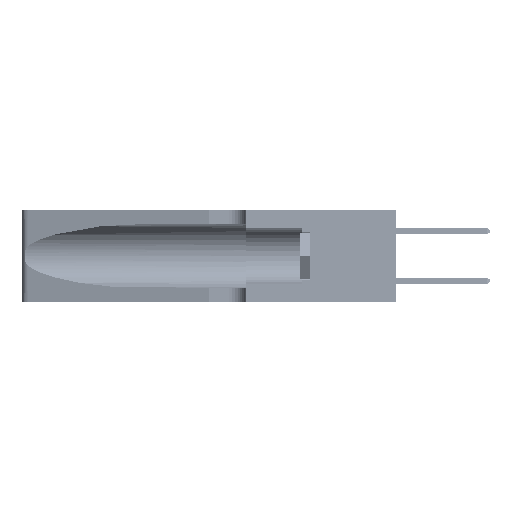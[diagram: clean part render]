
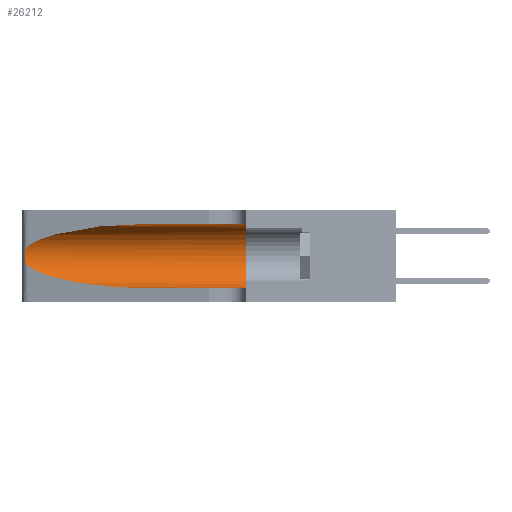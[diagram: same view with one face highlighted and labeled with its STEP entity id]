
A CAD part, left-side view. The second image highlights one B-rep face of the part: STEP entity #26212.
In plain terms, the highlighted cylindrical face has radius 3.308 mm (diameter 6.617 mm), a partial arc.
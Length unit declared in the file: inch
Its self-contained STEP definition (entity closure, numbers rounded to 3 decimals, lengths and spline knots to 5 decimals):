
#1398 = VECTOR ( 'NONE', #6263, 39.37008 ) ;
#2077 = EDGE_CURVE ( 'NONE', #12493, #4181, #42501, .T. ) ;
#3473 = CARTESIAN_POINT ( 'NONE',  ( 0.25555, 1.22993, 0.14849 ) ) ;
#3520 = ORIENTED_EDGE ( 'NONE', *, *, #21434, .T. ) ;
#4000 = CARTESIAN_POINT ( 'NONE',  ( 0.1305, 1.61858, 0.31525 ) ) ;
#4181 = VERTEX_POINT ( 'NONE', #4936 ) ;
#4400 = CARTESIAN_POINT ( 'NONE',  ( 0.1305, 0.72297, 0.31525 ) ) ;
#4936 = CARTESIAN_POINT ( 'NONE',  ( 0.25487, 1.22718, 0.22369 ) ) ;
#6263 = DIRECTION ( 'NONE',  ( 0., -1., 0. ) ) ;
#6633 = CARTESIAN_POINT ( 'NONE',  ( 0.1305, 1.61858, 0.185 ) ) ;
#6638 = CARTESIAN_POINT ( 'NONE',  ( 0.1305, 0.35, 0.185 ) ) ;
#7102 = AXIS2_PLACEMENT_3D ( 'NONE', #6633, #22961, #48681 ) ;
#7197 = CARTESIAN_POINT ( 'NONE',  ( 0.25854, 1.2359, 0.20912 ) ) ;
#7915 = CARTESIAN_POINT ( 'NONE',  ( 0.26075, 1.23896, 0.19203 ) ) ;
#11277 = CARTESIAN_POINT ( 'NONE',  ( 0.25789, 1.23486, 0.15765 ) ) ;
#11459 = DIRECTION ( 'NONE',  ( 0., -1., 0. ) ) ;
#12394 = AXIS2_PLACEMENT_3D ( 'NONE', #6638, #47275, #43698 ) ;
#12493 = VERTEX_POINT ( 'NONE', #41396 ) ;
#13958 = ORIENTED_EDGE ( 'NONE', *, *, #43957, .F. ) ;
#14620 = ORIENTED_EDGE ( 'NONE', *, *, #49664, .T. ) ;
#15398 = CARTESIAN_POINT ( 'NONE',  ( 0.25487, 1.22718, 0.14631 ) ) ;
#16158 = CARTESIAN_POINT ( 'NONE',  ( 0.2373, 1.15595, 0.28018 ) ) ;
#17265 = LINE ( 'NONE', #4000, #48566 ) ;
#17450 = CARTESIAN_POINT ( 'NONE',  ( 0.1305, 0.72297, 0.05475 ) ) ;
#18318 = CARTESIAN_POINT ( 'NONE',  ( 0.1305, 1.61858, 0.05475 ) ) ;
#18928 = VERTEX_POINT ( 'NONE', #27120 ) ;
#19602 = CARTESIAN_POINT ( 'NONE',  ( 0.25555, 1.22994, 0.2215 ) ) ;
#20443 = ORIENTED_EDGE ( 'NONE', *, *, #52382, .F. ) ;
#20881 = B_SPLINE_CURVE_WITH_KNOTS ( 'NONE', 3,
 ( #48020, #19602, #52077, #36046, #7197, #32284, #7915, #36410, #48202, #23694, #11277, #39815, #3473, #15398 ),
 .UNSPECIFIED., .F., .F.,
 ( 4, 2, 2, 2, 2, 2, 4 ),
 ( 0., 0.00027, 0.00053, 0.00107, 0.0016, 0.00187, 0.00214 ),
 .UNSPECIFIED. ) ;
#21434 = EDGE_CURVE ( 'NONE', #4181, #32012, #20881, .T. ) ;
#22961 = DIRECTION ( 'NONE',  ( 0., -1., 0. ) ) ;
#23694 = CARTESIAN_POINT ( 'NONE',  ( 0.25856, 1.23593, 0.16098 ) ) ;
#24824 = ORIENTED_EDGE ( 'NONE', *, *, #2077, .T. ) ;
#24827 = CIRCLE ( 'NONE', #12394, 0.13025 ) ;
#25618 = CARTESIAN_POINT ( 'NONE',  ( 0.1305, 0.35, 0.31525 ) ) ;
#26212 = ADVANCED_FACE ( 'NONE', ( #35969 ), #43005, .F. ) ;
#27120 = CARTESIAN_POINT ( 'NONE',  ( 0.1305, 0.72297, 0.05475 ) ) ;
#27376 = CARTESIAN_POINT ( 'NONE',  ( 0.25487, 1.22718, 0.14631 ) ) ;
#28556 = CARTESIAN_POINT ( 'NONE',  ( 0.18966, 0.96281, 0.31525 ) ) ;
#29358 = CARTESIAN_POINT ( 'NONE',  ( 0.18966, 0.96281, 0.05475 ) ) ;
#32012 = VERTEX_POINT ( 'NONE', #27376 ) ;
#32284 = CARTESIAN_POINT ( 'NONE',  ( 0.26018, 1.23835, 0.19895 ) ) ;
#35085 = EDGE_LOOP ( 'NONE', ( #24824, #3520, #14620, #39989, #13958, #20443 ) ) ;
#35969 = FACE_OUTER_BOUND ( 'NONE', #35085, .T. ) ;
#36046 = CARTESIAN_POINT ( 'NONE',  ( 0.25787, 1.23484, 0.2124 ) ) ;
#36410 = CARTESIAN_POINT ( 'NONE',  ( 0.26075, 1.23896, 0.178 ) ) ;
#36618 = CARTESIAN_POINT ( 'NONE',  ( 0.1305, 0.35, 0.05475 ) ) ;
#36928 =( BOUNDED_CURVE ( )  B_SPLINE_CURVE ( 3, ( #45468, #41922, #29358, #17450 ),
 .UNSPECIFIED., .F., .T. ) 
 B_SPLINE_CURVE_WITH_KNOTS ( ( 4, 4 ),
 ( 3.44316, 4.71239 ),
 .UNSPECIFIED. ) 
 CURVE ( )  GEOMETRIC_REPRESENTATION_ITEM ( )  RATIONAL_B_SPLINE_CURVE ( ( 1., 0.87, 0.87, 1. ) ) 
 REPRESENTATION_ITEM ( '' )  );
#39815 = CARTESIAN_POINT ( 'NONE',  ( 0.25639, 1.23186, 0.15144 ) ) ;
#39989 = ORIENTED_EDGE ( 'NONE', *, *, #47511, .T. ) ;
#41396 = CARTESIAN_POINT ( 'NONE',  ( 0.1305, 0.72297, 0.31525 ) ) ;
#41922 = CARTESIAN_POINT ( 'NONE',  ( 0.2373, 1.15595, 0.08982 ) ) ;
#42501 =( BOUNDED_CURVE ( )  B_SPLINE_CURVE ( 3, ( #4400, #28556, #16158, #45032 ),
 .UNSPECIFIED., .F., .F. ) 
 B_SPLINE_CURVE_WITH_KNOTS ( ( 4, 4 ),
 ( 1.5708, 2.84003 ),
 .UNSPECIFIED. ) 
 CURVE ( )  GEOMETRIC_REPRESENTATION_ITEM ( )  RATIONAL_B_SPLINE_CURVE ( ( 1., 0.87, 0.87, 1. ) ) 
 REPRESENTATION_ITEM ( '' )  );
#43005 = CYLINDRICAL_SURFACE ( 'NONE', #7102, 0.13025 ) ;
#43463 = LINE ( 'NONE', #18318, #1398 ) ;
#43698 = DIRECTION ( 'NONE',  ( 0., 0., 1. ) ) ;
#43957 = EDGE_CURVE ( 'NONE', #49707, #46626, #24827, .T. ) ;
#45032 = CARTESIAN_POINT ( 'NONE',  ( 0.25487, 1.22718, 0.22369 ) ) ;
#45468 = CARTESIAN_POINT ( 'NONE',  ( 0.25487, 1.22718, 0.14631 ) ) ;
#46626 = VERTEX_POINT ( 'NONE', #36618 ) ;
#47275 = DIRECTION ( 'NONE',  ( 0., 1., 0. ) ) ;
#47511 = EDGE_CURVE ( 'NONE', #18928, #46626, #43463, .T. ) ;
#48020 = CARTESIAN_POINT ( 'NONE',  ( 0.25487, 1.22718, 0.22369 ) ) ;
#48202 = CARTESIAN_POINT ( 'NONE',  ( 0.26017, 1.23833, 0.17102 ) ) ;
#48566 = VECTOR ( 'NONE', #11459, 39.37008 ) ;
#48681 = DIRECTION ( 'NONE',  ( 0., 0., -1. ) ) ;
#49664 = EDGE_CURVE ( 'NONE', #32012, #18928, #36928, .T. ) ;
#49707 = VERTEX_POINT ( 'NONE', #25618 ) ;
#52077 = CARTESIAN_POINT ( 'NONE',  ( 0.25639, 1.23184, 0.21858 ) ) ;
#52382 = EDGE_CURVE ( 'NONE', #12493, #49707, #17265, .T. ) ;
